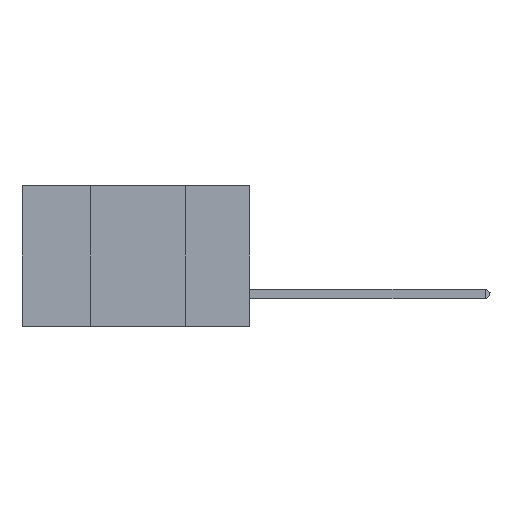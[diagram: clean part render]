
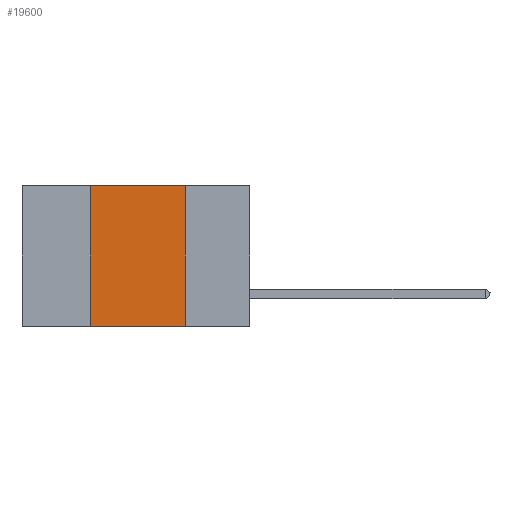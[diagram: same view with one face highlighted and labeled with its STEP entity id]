
A CAD part, left-side view. The second image highlights one B-rep face of the part: STEP entity #19600.
In plain terms, the highlighted planar face has unit normal (-1, 0, 0).
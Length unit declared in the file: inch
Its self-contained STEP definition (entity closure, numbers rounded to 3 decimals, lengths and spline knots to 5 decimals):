
#416 = CARTESIAN_POINT ( 'NONE',  ( 0., 0.6, 0. ) ) ;
#1521 = DIRECTION ( 'NONE',  ( 0., -1., 0. ) ) ;
#3080 = CARTESIAN_POINT ( 'NONE',  ( 0., 0.17, -0.37 ) ) ;
#3761 = CARTESIAN_POINT ( 'NONE',  ( 0., 0.6, -0.37 ) ) ;
#4515 = LINE ( 'NONE', #416, #21085 ) ;
#6354 = CARTESIAN_POINT ( 'NONE',  ( 0., 0.42, -0.37 ) ) ;
#7534 = DIRECTION ( 'NONE',  ( 1., 0., 0. ) ) ;
#9295 = LINE ( 'NONE', #29582, #23106 ) ;
#9971 = AXIS2_PLACEMENT_3D ( 'NONE', #22276, #7534, #12326 ) ;
#10095 = DIRECTION ( 'NONE',  ( 0., -1., 0. ) ) ;
#10601 = VECTOR ( 'NONE', #1521, 39.37008 ) ;
#12167 = VERTEX_POINT ( 'NONE', #19289 ) ;
#12326 = DIRECTION ( 'NONE',  ( 0., 0., -1. ) ) ;
#13016 = LINE ( 'NONE', #21257, #21860 ) ;
#14048 = ORIENTED_EDGE ( 'NONE', *, *, #26559, .F. ) ;
#14807 = PLANE ( 'NONE',  #9971 ) ;
#14944 = EDGE_LOOP ( 'NONE', ( #19586, #23010, #14048, #19235 ) ) ;
#16764 = VERTEX_POINT ( 'NONE', #30251 ) ;
#19235 = ORIENTED_EDGE ( 'NONE', *, *, #27964, .T. ) ;
#19289 = CARTESIAN_POINT ( 'NONE',  ( 0., 0.17, 0. ) ) ;
#19586 = ORIENTED_EDGE ( 'NONE', *, *, #19642, .F. ) ;
#19600 = ADVANCED_FACE ( 'NONE', ( #30685 ), #14807, .F. ) ;
#19642 = EDGE_CURVE ( 'NONE', #12167, #22610, #9295, .T. ) ;
#21085 = VECTOR ( 'NONE', #10095, 39.37008 ) ;
#21257 = CARTESIAN_POINT ( 'NONE',  ( 0., 0.42, 0. ) ) ;
#21860 = VECTOR ( 'NONE', #31084, 39.37008 ) ;
#22276 = CARTESIAN_POINT ( 'NONE',  ( 0., 0.6, 0. ) ) ;
#22392 = DIRECTION ( 'NONE',  ( 0., 0., -1. ) ) ;
#22610 = VERTEX_POINT ( 'NONE', #3080 ) ;
#23010 = ORIENTED_EDGE ( 'NONE', *, *, #26777, .F. ) ;
#23106 = VECTOR ( 'NONE', #22392, 39.37008 ) ;
#26559 = EDGE_CURVE ( 'NONE', #29753, #16764, #13016, .T. ) ;
#26777 = EDGE_CURVE ( 'NONE', #16764, #12167, #4515, .T. ) ;
#27033 = LINE ( 'NONE', #3761, #10601 ) ;
#27964 = EDGE_CURVE ( 'NONE', #29753, #22610, #27033, .T. ) ;
#29582 = CARTESIAN_POINT ( 'NONE',  ( 0., 0.17, 0. ) ) ;
#29753 = VERTEX_POINT ( 'NONE', #6354 ) ;
#30251 = CARTESIAN_POINT ( 'NONE',  ( 0., 0.42, 0. ) ) ;
#30685 = FACE_OUTER_BOUND ( 'NONE', #14944, .T. ) ;
#31084 = DIRECTION ( 'NONE',  ( 0., 0., 1. ) ) ;
